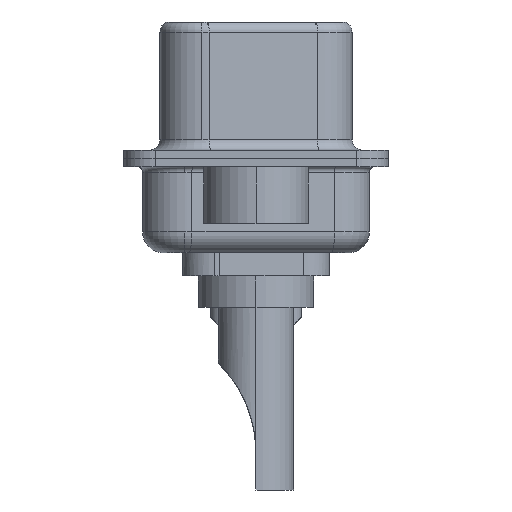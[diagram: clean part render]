
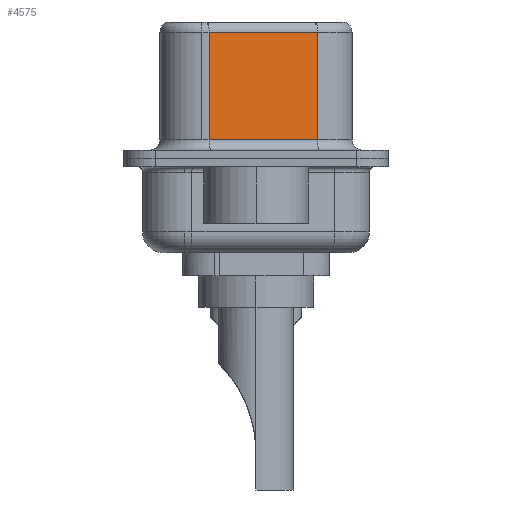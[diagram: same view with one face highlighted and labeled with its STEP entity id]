
A CAD part, left-side view. The second image highlights one B-rep face of the part: STEP entity #4575.
In plain terms, the highlighted planar face has unit normal (-0.985, -0.174, 0).
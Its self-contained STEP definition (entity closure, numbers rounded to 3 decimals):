
#1002 = LINE ( 'NONE', #3800, #6522 ) ;
#1717 = EDGE_CURVE ( 'NONE', #4727, #1891, #1002, .T. ) ;
#1891 = VERTEX_POINT ( 'NONE', #5728 ) ;
#2959 = VECTOR ( 'NONE', #24510, 1000. ) ;
#3800 = CARTESIAN_POINT ( 'NONE',  ( 4.58, -2.927, 6.52 ) ) ;
#3960 = EDGE_CURVE ( 'NONE', #4727, #22763, #11542, .T. ) ;
#4575 = ADVANCED_FACE ( 'NONE', ( #5853 ), #24813, .F. ) ;
#4727 = VERTEX_POINT ( 'NONE', #8736 ) ;
#4837 = EDGE_CURVE ( 'NONE', #22763, #10783, #22905, .T. ) ;
#5416 = ORIENTED_EDGE ( 'NONE', *, *, #4837, .T. ) ;
#5728 = CARTESIAN_POINT ( 'NONE',  ( 4.58, -2.927, 0.9 ) ) ;
#5853 = FACE_OUTER_BOUND ( 'NONE', #14580, .T. ) ;
#5986 = LINE ( 'NONE', #8946, #15385 ) ;
#6522 = VECTOR ( 'NONE', #18694, 1000. ) ;
#8736 = CARTESIAN_POINT ( 'NONE',  ( 4.58, -2.927, 6.02 ) ) ;
#8946 = CARTESIAN_POINT ( 'NONE',  ( 4.58, -2.927, 0.9 ) ) ;
#9911 = EDGE_CURVE ( 'NONE', #10783, #1891, #5986, .T. ) ;
#10265 = CARTESIAN_POINT ( 'NONE',  ( 3.67, 2.233, 6.02 ) ) ;
#10783 = VERTEX_POINT ( 'NONE', #23100 ) ;
#11407 = ORIENTED_EDGE ( 'NONE', *, *, #3960, .T. ) ;
#11542 = LINE ( 'NONE', #21161, #2959 ) ;
#14580 = EDGE_LOOP ( 'NONE', ( #14842, #11407, #5416, #26317 ) ) ;
#14646 = DIRECTION ( 'NONE',  ( 0., 0., -1. ) ) ;
#14842 = ORIENTED_EDGE ( 'NONE', *, *, #1717, .F. ) ;
#15385 = VECTOR ( 'NONE', #21030, 1000. ) ;
#15782 = AXIS2_PLACEMENT_3D ( 'NONE', #22117, #18936, #19366 ) ;
#16677 = CARTESIAN_POINT ( 'NONE',  ( 3.67, 2.233, 6.52 ) ) ;
#18694 = DIRECTION ( 'NONE',  ( 0., 0., -1. ) ) ;
#18757 = VECTOR ( 'NONE', #14646, 1000. ) ;
#18936 = DIRECTION ( 'NONE',  ( 0.985, 0.174, 0. ) ) ;
#19366 = DIRECTION ( 'NONE',  ( -0.174, 0.985, 0. ) ) ;
#21030 = DIRECTION ( 'NONE',  ( 0.174, -0.985, 0. ) ) ;
#21161 = CARTESIAN_POINT ( 'NONE',  ( 4.58, -2.927, 6.02 ) ) ;
#22117 = CARTESIAN_POINT ( 'NONE',  ( 4.58, -2.927, 6.52 ) ) ;
#22763 = VERTEX_POINT ( 'NONE', #10265 ) ;
#22905 = LINE ( 'NONE', #16677, #18757 ) ;
#23100 = CARTESIAN_POINT ( 'NONE',  ( 3.67, 2.233, 0.9 ) ) ;
#24510 = DIRECTION ( 'NONE',  ( -0.174, 0.985, 0. ) ) ;
#24813 = PLANE ( 'NONE',  #15782 ) ;
#26317 = ORIENTED_EDGE ( 'NONE', *, *, #9911, .T. ) ;
